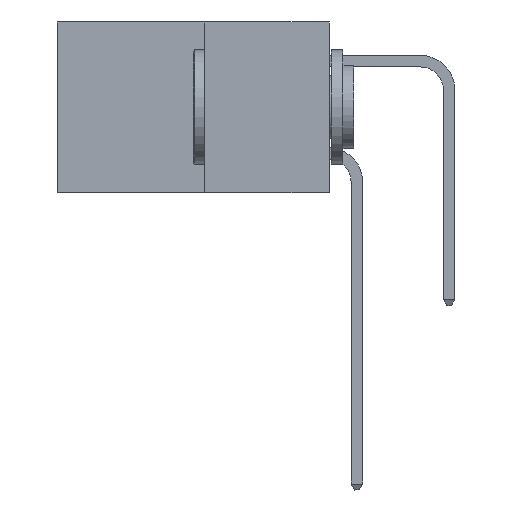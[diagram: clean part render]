
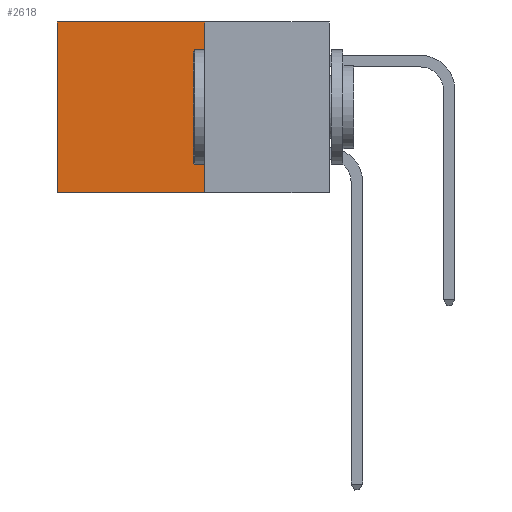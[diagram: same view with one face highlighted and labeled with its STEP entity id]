
A CAD part, left-side view. The second image highlights one B-rep face of the part: STEP entity #2618.
In plain terms, the highlighted planar face has unit normal (-1, 0, 0).
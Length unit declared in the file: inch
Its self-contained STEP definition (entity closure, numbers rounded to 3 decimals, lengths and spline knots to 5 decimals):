
#548 = DIRECTION ( 'NONE',  ( 1., 0., 0. ) ) ;
#1649 = DIRECTION ( 'NONE',  ( 0., 1., 0. ) ) ;
#1719 = CARTESIAN_POINT ( 'NONE',  ( 0.277, 0.27, -0.37 ) ) ;
#1868 = DIRECTION ( 'NONE',  ( 0., 0., -1. ) ) ;
#1976 = DIRECTION ( 'NONE',  ( 0., 1., 0. ) ) ;
#2562 = ORIENTED_EDGE ( 'NONE', *, *, #14892, .T. ) ;
#2618 = ADVANCED_FACE ( 'NONE', ( #26246 ), #31462, .F. ) ;
#3594 = CARTESIAN_POINT ( 'NONE',  ( 0.277, 0.27, -0.37 ) ) ;
#6443 = VECTOR ( 'NONE', #1976, 39.37008 ) ;
#6853 = LINE ( 'NONE', #31156, #19110 ) ;
#7888 = VECTOR ( 'NONE', #23921, 39.37008 ) ;
#8593 = EDGE_CURVE ( 'NONE', #23455, #17242, #25970, .T. ) ;
#12461 = CARTESIAN_POINT ( 'NONE',  ( 0.277, 0.59, 0. ) ) ;
#12877 = EDGE_CURVE ( 'NONE', #13706, #20071, #6853, .T. ) ;
#13483 = CARTESIAN_POINT ( 'NONE',  ( 0.277, 0.59, -0.37 ) ) ;
#13706 = VERTEX_POINT ( 'NONE', #22131 ) ;
#14892 = EDGE_CURVE ( 'NONE', #20071, #17242, #28144, .T. ) ;
#15007 = ORIENTED_EDGE ( 'NONE', *, *, #23368, .F. ) ;
#16636 = CARTESIAN_POINT ( 'NONE',  ( 0.277, 0.59, -0.37 ) ) ;
#17242 = VERTEX_POINT ( 'NONE', #13483 ) ;
#18070 = VECTOR ( 'NONE', #23405, 39.37008 ) ;
#19110 = VECTOR ( 'NONE', #1649, 39.37008 ) ;
#19382 = AXIS2_PLACEMENT_3D ( 'NONE', #1719, #548, #1868 ) ;
#20071 = VERTEX_POINT ( 'NONE', #12461 ) ;
#20970 = CARTESIAN_POINT ( 'NONE',  ( 0.277, 0.27, -0.37 ) ) ;
#21169 = CARTESIAN_POINT ( 'NONE',  ( 0.277, 0.27, -0.37 ) ) ;
#21437 = ORIENTED_EDGE ( 'NONE', *, *, #8593, .F. ) ;
#22131 = CARTESIAN_POINT ( 'NONE',  ( 0.277, 0.27, 0. ) ) ;
#23368 = EDGE_CURVE ( 'NONE', #13706, #23455, #30997, .T. ) ;
#23405 = DIRECTION ( 'NONE',  ( 0., 0., -1. ) ) ;
#23455 = VERTEX_POINT ( 'NONE', #21169 ) ;
#23921 = DIRECTION ( 'NONE',  ( 0., 0., -1. ) ) ;
#25970 = LINE ( 'NONE', #3594, #6443 ) ;
#26246 = FACE_OUTER_BOUND ( 'NONE', #28439, .T. ) ;
#28144 = LINE ( 'NONE', #16636, #7888 ) ;
#28439 = EDGE_LOOP ( 'NONE', ( #2562, #21437, #15007, #30099 ) ) ;
#30099 = ORIENTED_EDGE ( 'NONE', *, *, #12877, .T. ) ;
#30997 = LINE ( 'NONE', #20970, #18070 ) ;
#31156 = CARTESIAN_POINT ( 'NONE',  ( 0.277, 0.27, 0. ) ) ;
#31462 = PLANE ( 'NONE',  #19382 ) ;
